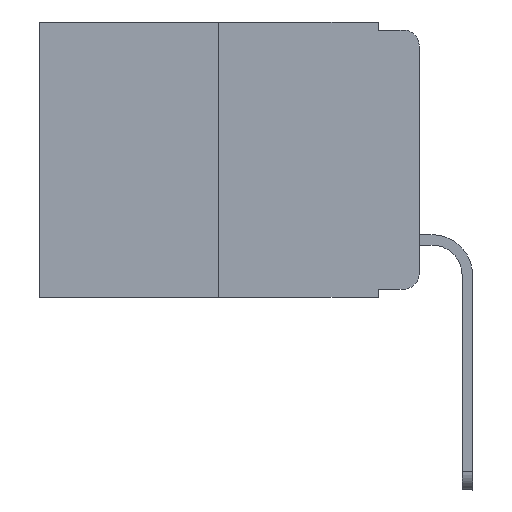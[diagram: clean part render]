
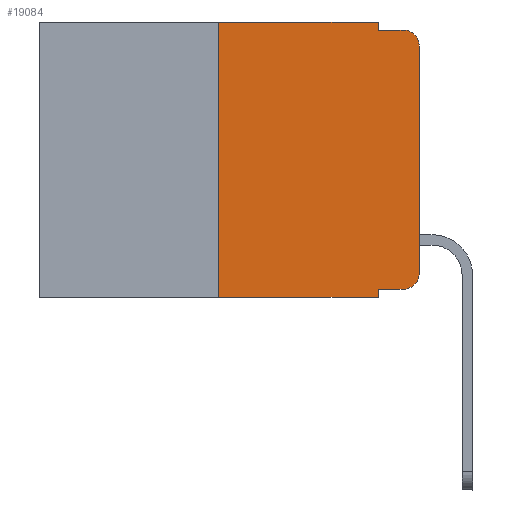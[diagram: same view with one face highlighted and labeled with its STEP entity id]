
A CAD part, left-side view. The second image highlights one B-rep face of the part: STEP entity #19084.
In plain terms, the highlighted planar face has unit normal (-1, 0, 0).
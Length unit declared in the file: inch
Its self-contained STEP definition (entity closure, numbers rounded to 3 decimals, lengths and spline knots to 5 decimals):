
#98 = DIRECTION ( 'NONE',  ( 0., -1., 0. ) ) ;
#222 = DIRECTION ( 'NONE',  ( 0., 0., -1. ) ) ;
#422 = DIRECTION ( 'NONE',  ( 1., 0., 0. ) ) ;
#576 = CARTESIAN_POINT ( 'NONE',  ( 0., 0.051, -0.343 ) ) ;
#770 = DIRECTION ( 'NONE',  ( 0., 0., -1. ) ) ;
#784 = ORIENTED_EDGE ( 'NONE', *, *, #6380, .T. ) ;
#1137 = CARTESIAN_POINT ( 'NONE',  ( 0., 0., 0. ) ) ;
#1809 = VECTOR ( 'NONE', #7850, 39.37008 ) ;
#1867 = CARTESIAN_POINT ( 'NONE',  ( 0., 0., -0.03 ) ) ;
#2086 = VECTOR ( 'NONE', #20940, 39.37008 ) ;
#2486 = CARTESIAN_POINT ( 'NONE',  ( 0., 0.051, 0. ) ) ;
#2898 = CARTESIAN_POINT ( 'NONE',  ( 0., 0.25, 0. ) ) ;
#2929 = VERTEX_POINT ( 'NONE', #19444 ) ;
#3114 = CARTESIAN_POINT ( 'NONE',  ( 0., 0., -0.313 ) ) ;
#3204 = AXIS2_PLACEMENT_3D ( 'NONE', #11178, #422, #770 ) ;
#3962 = VERTEX_POINT ( 'NONE', #2486 ) ;
#4215 = VECTOR ( 'NONE', #222, 39.37008 ) ;
#4394 = VECTOR ( 'NONE', #21276, 39.37008 ) ;
#4455 = DIRECTION ( 'NONE',  ( 0., 0., -1. ) ) ;
#4572 = CARTESIAN_POINT ( 'NONE',  ( 0., 0.02, -0.313 ) ) ;
#4648 = EDGE_CURVE ( 'NONE', #2929, #6693, #17398, .T. ) ;
#4742 = CIRCLE ( 'NONE', #20794, 0.02 ) ;
#5395 = ORIENTED_EDGE ( 'NONE', *, *, #8356, .F. ) ;
#5781 = DIRECTION ( 'NONE',  ( 0., -1., 0. ) ) ;
#6205 = ORIENTED_EDGE ( 'NONE', *, *, #4648, .F. ) ;
#6380 = EDGE_CURVE ( 'NONE', #7810, #10383, #22414, .T. ) ;
#6438 = CARTESIAN_POINT ( 'NONE',  ( 0., 0.051, 0. ) ) ;
#6518 = EDGE_CURVE ( 'NONE', #10383, #21024, #13700, .T. ) ;
#6693 = VERTEX_POINT ( 'NONE', #2898 ) ;
#7078 = CARTESIAN_POINT ( 'NONE',  ( 0., 0.051, -0.333 ) ) ;
#7292 = EDGE_CURVE ( 'NONE', #11532, #8692, #17472, .T. ) ;
#7532 = CARTESIAN_POINT ( 'NONE',  ( 0., 0.02, -0.333 ) ) ;
#7810 = VERTEX_POINT ( 'NONE', #7532 ) ;
#7850 = DIRECTION ( 'NONE',  ( 0., 0., -1. ) ) ;
#8067 = LINE ( 'NONE', #6438, #1809 ) ;
#8356 = EDGE_CURVE ( 'NONE', #3962, #13486, #8067, .T. ) ;
#8492 = VECTOR ( 'NONE', #5781, 39.37008 ) ;
#8692 = VERTEX_POINT ( 'NONE', #576 ) ;
#8730 = DIRECTION ( 'NONE',  ( 0., 0., -1. ) ) ;
#8940 = VECTOR ( 'NONE', #10164, 39.37008 ) ;
#9307 = AXIS2_PLACEMENT_3D ( 'NONE', #4572, #21479, #4455 ) ;
#10164 = DIRECTION ( 'NONE',  ( 0., 0., 1. ) ) ;
#10338 = CARTESIAN_POINT ( 'NONE',  ( 0., 0.051, -0.01 ) ) ;
#10383 = VERTEX_POINT ( 'NONE', #3114 ) ;
#10533 = CARTESIAN_POINT ( 'NONE',  ( 0., 0.25, 0. ) ) ;
#10658 = LINE ( 'NONE', #10338, #13204 ) ;
#10840 = EDGE_CURVE ( 'NONE', #2929, #8692, #11274, .T. ) ;
#11067 = PLANE ( 'NONE',  #3204 ) ;
#11178 = CARTESIAN_POINT ( 'NONE',  ( 0., 0.473, 0. ) ) ;
#11274 = LINE ( 'NONE', #19616, #8492 ) ;
#11282 = CARTESIAN_POINT ( 'NONE',  ( 0., 0.051, -0.01 ) ) ;
#11532 = VERTEX_POINT ( 'NONE', #11899 ) ;
#11878 = EDGE_LOOP ( 'NONE', ( #17782, #12731, #18394, #5395, #22502, #6205, #17726, #16212, #18287, #784 ) ) ;
#11899 = CARTESIAN_POINT ( 'NONE',  ( 0., 0.051, -0.333 ) ) ;
#12657 = LINE ( 'NONE', #7078, #16917 ) ;
#12731 = ORIENTED_EDGE ( 'NONE', *, *, #19798, .T. ) ;
#12834 = CARTESIAN_POINT ( 'NONE',  ( 0., 0.02, -0.01 ) ) ;
#13204 = VECTOR ( 'NONE', #21281, 39.37008 ) ;
#13334 = EDGE_CURVE ( 'NONE', #11532, #7810, #12657, .T. ) ;
#13486 = VERTEX_POINT ( 'NONE', #11282 ) ;
#13700 = LINE ( 'NONE', #1137, #8940 ) ;
#13965 = CARTESIAN_POINT ( 'NONE',  ( 0., 0.473, 0. ) ) ;
#14082 = EDGE_CURVE ( 'NONE', #13486, #14285, #10658, .T. ) ;
#14285 = VERTEX_POINT ( 'NONE', #12834 ) ;
#15464 = LINE ( 'NONE', #13965, #2086 ) ;
#15482 = DIRECTION ( 'NONE',  ( -1., 0., 0. ) ) ;
#16212 = ORIENTED_EDGE ( 'NONE', *, *, #7292, .F. ) ;
#16917 = VECTOR ( 'NONE', #98, 39.37008 ) ;
#17167 = CARTESIAN_POINT ( 'NONE',  ( 0., 0.02, -0.03 ) ) ;
#17398 = LINE ( 'NONE', #10533, #4394 ) ;
#17472 = LINE ( 'NONE', #19099, #4215 ) ;
#17726 = ORIENTED_EDGE ( 'NONE', *, *, #10840, .T. ) ;
#17782 = ORIENTED_EDGE ( 'NONE', *, *, #6518, .T. ) ;
#18287 = ORIENTED_EDGE ( 'NONE', *, *, #13334, .T. ) ;
#18394 = ORIENTED_EDGE ( 'NONE', *, *, #14082, .F. ) ;
#18745 = EDGE_CURVE ( 'NONE', #6693, #3962, #15464, .T. ) ;
#19084 = ADVANCED_FACE ( 'NONE', ( #19740 ), #11067, .F. ) ;
#19099 = CARTESIAN_POINT ( 'NONE',  ( 0., 0.051, 0. ) ) ;
#19444 = CARTESIAN_POINT ( 'NONE',  ( 0., 0.25, -0.343 ) ) ;
#19616 = CARTESIAN_POINT ( 'NONE',  ( 0., 0.473, -0.343 ) ) ;
#19740 = FACE_OUTER_BOUND ( 'NONE', #11878, .T. ) ;
#19798 = EDGE_CURVE ( 'NONE', #21024, #14285, #4742, .T. ) ;
#20794 = AXIS2_PLACEMENT_3D ( 'NONE', #17167, #15482, #8730 ) ;
#20940 = DIRECTION ( 'NONE',  ( 0., -1., 0. ) ) ;
#21024 = VERTEX_POINT ( 'NONE', #1867 ) ;
#21276 = DIRECTION ( 'NONE',  ( 0., 0., 1. ) ) ;
#21281 = DIRECTION ( 'NONE',  ( 0., -1., 0. ) ) ;
#21479 = DIRECTION ( 'NONE',  ( -1., 0., 0. ) ) ;
#22414 = CIRCLE ( 'NONE', #9307, 0.02 ) ;
#22502 = ORIENTED_EDGE ( 'NONE', *, *, #18745, .F. ) ;
